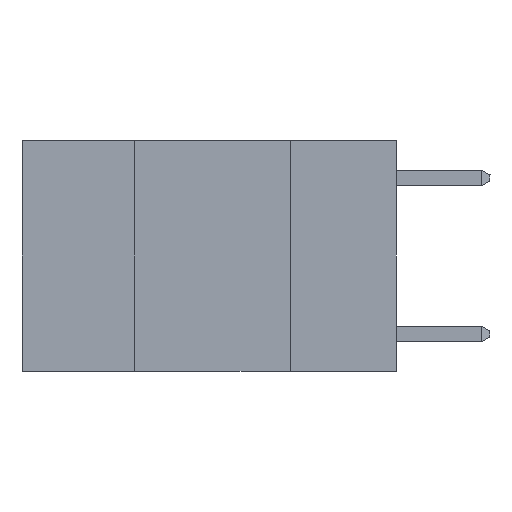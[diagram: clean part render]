
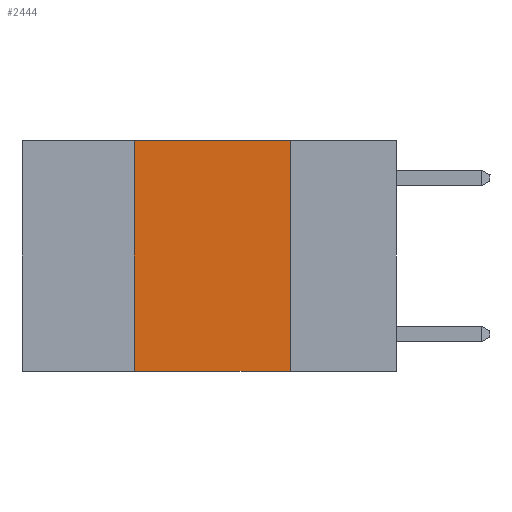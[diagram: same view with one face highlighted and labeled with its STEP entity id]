
A CAD part, left-side view. The second image highlights one B-rep face of the part: STEP entity #2444.
In plain terms, the highlighted planar face has unit normal (-1, 0, 0).
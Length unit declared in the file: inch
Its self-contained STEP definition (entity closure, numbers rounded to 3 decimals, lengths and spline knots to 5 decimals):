
#60 = LINE ( 'NONE', #6851, #4554 ) ;
#206 = CARTESIAN_POINT ( 'NONE',  ( 0., 0.17, 0. ) ) ;
#309 = DIRECTION ( 'NONE',  ( 0., 0., -1. ) ) ;
#912 = LINE ( 'NONE', #6384, #6203 ) ;
#995 = FACE_OUTER_BOUND ( 'NONE', #8143, .T. ) ;
#1002 = LINE ( 'NONE', #5790, #5661 ) ;
#1451 = ORIENTED_EDGE ( 'NONE', *, *, #6724, .T. ) ;
#1536 = CARTESIAN_POINT ( 'NONE',  ( 0., 0.42, 0. ) ) ;
#2444 = ADVANCED_FACE ( 'NONE', ( #995 ), #3035, .F. ) ;
#2462 = CARTESIAN_POINT ( 'NONE',  ( 0., 0.42, -0.37 ) ) ;
#3035 = PLANE ( 'NONE',  #5120 ) ;
#3080 = CARTESIAN_POINT ( 'NONE',  ( 0., 0.17, 0. ) ) ;
#3320 = VECTOR ( 'NONE', #5730, 39.37008 ) ;
#3533 = VERTEX_POINT ( 'NONE', #206 ) ;
#3606 = EDGE_CURVE ( 'NONE', #3709, #8389, #912, .T. ) ;
#3709 = VERTEX_POINT ( 'NONE', #2462 ) ;
#3731 = CARTESIAN_POINT ( 'NONE',  ( 0., 0.6, 0. ) ) ;
#4554 = VECTOR ( 'NONE', #4709, 39.37008 ) ;
#4709 = DIRECTION ( 'NONE',  ( 0., -1., 0. ) ) ;
#4891 = VERTEX_POINT ( 'NONE', #6425 ) ;
#5051 = DIRECTION ( 'NONE',  ( 0., 0., 1. ) ) ;
#5120 = AXIS2_PLACEMENT_3D ( 'NONE', #3731, #6443, #309 ) ;
#5132 = DIRECTION ( 'NONE',  ( 0., -1., 0. ) ) ;
#5661 = VECTOR ( 'NONE', #5132, 39.37008 ) ;
#5730 = DIRECTION ( 'NONE',  ( 0., 0., -1. ) ) ;
#5751 = ORIENTED_EDGE ( 'NONE', *, *, #8530, .F. ) ;
#5790 = CARTESIAN_POINT ( 'NONE',  ( 0., 0.6, 0. ) ) ;
#5912 = LINE ( 'NONE', #3080, #3320 ) ;
#6203 = VECTOR ( 'NONE', #5051, 39.37008 ) ;
#6384 = CARTESIAN_POINT ( 'NONE',  ( 0., 0.42, 0. ) ) ;
#6425 = CARTESIAN_POINT ( 'NONE',  ( 0., 0.17, -0.37 ) ) ;
#6443 = DIRECTION ( 'NONE',  ( 1., 0., 0. ) ) ;
#6724 = EDGE_CURVE ( 'NONE', #3709, #4891, #60, .T. ) ;
#6851 = CARTESIAN_POINT ( 'NONE',  ( 0., 0.6, -0.37 ) ) ;
#7304 = ORIENTED_EDGE ( 'NONE', *, *, #8045, .F. ) ;
#8045 = EDGE_CURVE ( 'NONE', #8389, #3533, #1002, .T. ) ;
#8143 = EDGE_LOOP ( 'NONE', ( #5751, #7304, #8654, #1451 ) ) ;
#8389 = VERTEX_POINT ( 'NONE', #1536 ) ;
#8530 = EDGE_CURVE ( 'NONE', #3533, #4891, #5912, .T. ) ;
#8654 = ORIENTED_EDGE ( 'NONE', *, *, #3606, .F. ) ;
